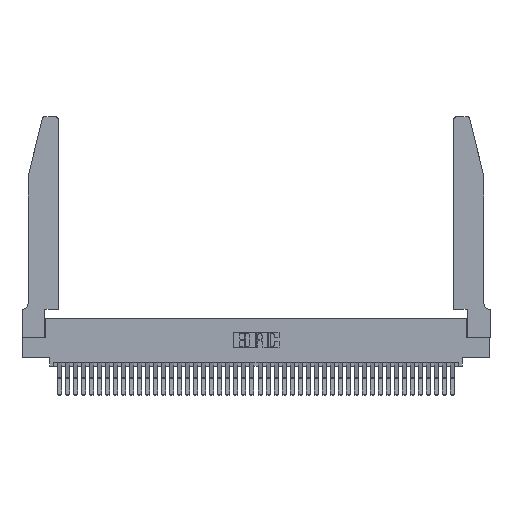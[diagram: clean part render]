
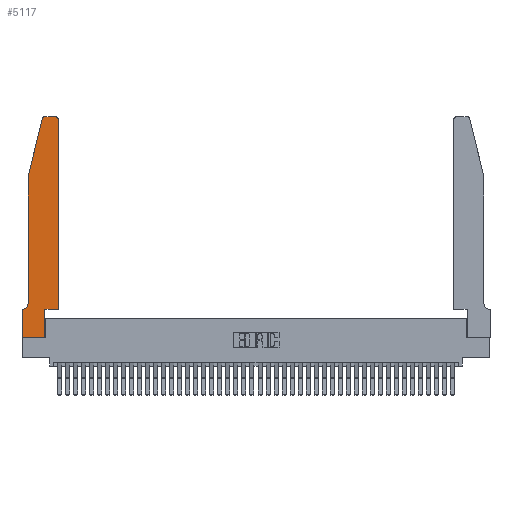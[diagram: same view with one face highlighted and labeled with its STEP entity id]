
A CAD part, top view. The second image highlights one B-rep face of the part: STEP entity #5117.
In plain terms, the highlighted planar face has unit normal (0, 0, 1).
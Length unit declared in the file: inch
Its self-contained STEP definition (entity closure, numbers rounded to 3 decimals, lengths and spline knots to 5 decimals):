
#58 = CARTESIAN_POINT ( 'NONE',  ( 0.0055, 0.42, 0.37 ) ) ;
#121 = EDGE_CURVE ( 'NONE', #27266, #37810, #22057, .T. ) ;
#180 = EDGE_CURVE ( 'NONE', #30962, #11434, #19940, .T. ) ;
#817 = DIRECTION ( 'NONE',  ( 1., 0., 0. ) ) ;
#1511 = ORIENTED_EDGE ( 'NONE', *, *, #180, .T. ) ;
#1961 = DIRECTION ( 'NONE',  ( 0., -1., 0. ) ) ;
#2182 = ORIENTED_EDGE ( 'NONE', *, *, #34164, .T. ) ;
#3515 = DIRECTION ( 'NONE',  ( -1., 0., 0. ) ) ;
#4806 = VECTOR ( 'NONE', #10750, 39.37008 ) ;
#5041 = LINE ( 'NONE', #36762, #21763 ) ;
#5117 = ADVANCED_FACE ( 'NONE', ( #43057 ), #40735, .T. ) ;
#5299 = ORIENTED_EDGE ( 'NONE', *, *, #14203, .T. ) ;
#5382 = CARTESIAN_POINT ( 'NONE',  ( 0., 0., 0.37 ) ) ;
#5452 = AXIS2_PLACEMENT_3D ( 'NONE', #30753, #20902, #817 ) ;
#6016 = VERTEX_POINT ( 'NONE', #10846 ) ;
#6853 = CARTESIAN_POINT ( 'NONE',  ( 0.0755, 2., 0.37 ) ) ;
#6960 = DIRECTION ( 'NONE',  ( 0., 0., 1. ) ) ;
#7307 = VECTOR ( 'NONE', #1961, 39.37008 ) ;
#7710 = VERTEX_POINT ( 'NONE', #37057 ) ;
#7961 = EDGE_CURVE ( 'NONE', #31423, #30962, #41799, .T. ) ;
#9518 = VECTOR ( 'NONE', #15072, 39.37008 ) ;
#9630 = EDGE_CURVE ( 'NONE', #13893, #27266, #41413, .T. ) ;
#10364 = CARTESIAN_POINT ( 'NONE',  ( 0., 0.35, 0.37 ) ) ;
#10545 = ORIENTED_EDGE ( 'NONE', *, *, #7961, .T. ) ;
#10750 = DIRECTION ( 'NONE',  ( 0., 1., 0. ) ) ;
#10846 = CARTESIAN_POINT ( 'NONE',  ( 0.0055, 0.35, 0.37 ) ) ;
#11434 = VERTEX_POINT ( 'NONE', #24727 ) ;
#11693 = CARTESIAN_POINT ( 'NONE',  ( 0.2865, 0., 0.37 ) ) ;
#11729 = CARTESIAN_POINT ( 'NONE',  ( 0.0755, 0.35, 0.37 ) ) ;
#11989 = DIRECTION ( 'NONE',  ( 0., 0., 1. ) ) ;
#12256 = EDGE_LOOP ( 'NONE', ( #35621, #10545, #1511, #38137, #2182, #19437, #5299, #24177, #23634, #24632, #42193, #20119 ) ) ;
#12315 = AXIS2_PLACEMENT_3D ( 'NONE', #58, #23558, #3515 ) ;
#12738 = EDGE_CURVE ( 'NONE', #6016, #31479, #36079, .T. ) ;
#13349 = VECTOR ( 'NONE', #40466, 39.37008 ) ;
#13879 = VECTOR ( 'NONE', #42275, 39.37008 ) ;
#13893 = VERTEX_POINT ( 'NONE', #40827 ) ;
#14203 = EDGE_CURVE ( 'NONE', #31479, #13893, #25088, .T. ) ;
#15072 = DIRECTION ( 'NONE',  ( -1., 0., 0. ) ) ;
#16356 = EDGE_CURVE ( 'NONE', #7710, #25746, #40161, .T. ) ;
#16581 = DIRECTION ( 'NONE',  ( 0., 1., 0. ) ) ;
#16738 = CARTESIAN_POINT ( 'NONE',  ( 0.284, 2.75, 0.37 ) ) ;
#16876 = DIRECTION ( 'NONE',  ( -0.239, -0.971, 0. ) ) ;
#19437 = ORIENTED_EDGE ( 'NONE', *, *, #12738, .T. ) ;
#19570 = CARTESIAN_POINT ( 'NONE',  ( 0.0755, 2., 0.37 ) ) ;
#19940 = LINE ( 'NONE', #6853, #27760 ) ;
#19994 = CARTESIAN_POINT ( 'NONE',  ( 0.2865, 0.35, 0.37 ) ) ;
#20119 = ORIENTED_EDGE ( 'NONE', *, *, #23086, .T. ) ;
#20258 = VERTEX_POINT ( 'NONE', #35682 ) ;
#20635 = CARTESIAN_POINT ( 'NONE',  ( 0.4505, 0.35, 0.37 ) ) ;
#20902 = DIRECTION ( 'NONE',  ( 0., 0., 1. ) ) ;
#21763 = VECTOR ( 'NONE', #40054, 39.37008 ) ;
#21783 = AXIS2_PLACEMENT_3D ( 'NONE', #31946, #11989, #35292 ) ;
#22057 = LINE ( 'NONE', #19994, #30847 ) ;
#22251 = VECTOR ( 'NONE', #26157, 39.37008 ) ;
#22292 = LINE ( 'NONE', #20635, #13349 ) ;
#23086 = EDGE_CURVE ( 'NONE', #25746, #31491, #33403, .T. ) ;
#23558 = DIRECTION ( 'NONE',  ( 0., 0., -1. ) ) ;
#23634 = ORIENTED_EDGE ( 'NONE', *, *, #121, .T. ) ;
#24177 = ORIENTED_EDGE ( 'NONE', *, *, #9630, .T. ) ;
#24349 = LINE ( 'NONE', #19570, #22251 ) ;
#24632 = ORIENTED_EDGE ( 'NONE', *, *, #37028, .T. ) ;
#24727 = CARTESIAN_POINT ( 'NONE',  ( 0.0755, 2., 0.37 ) ) ;
#25088 = LINE ( 'NONE', #5382, #7307 ) ;
#25746 = VERTEX_POINT ( 'NONE', #30775 ) ;
#26157 = DIRECTION ( 'NONE',  ( 0., -1., 0. ) ) ;
#26604 = CARTESIAN_POINT ( 'NONE',  ( 0.25487, 2.72718, 0.37 ) ) ;
#26967 = CARTESIAN_POINT ( 'NONE',  ( 0.4205, 2.72, 0.37 ) ) ;
#27266 = VERTEX_POINT ( 'NONE', #11693 ) ;
#27760 = VECTOR ( 'NONE', #16876, 39.37008 ) ;
#29004 = CARTESIAN_POINT ( 'NONE',  ( 0., 0., 0.37 ) ) ;
#30259 = DIRECTION ( 'NONE',  ( 1., 0., 0. ) ) ;
#30437 = CARTESIAN_POINT ( 'NONE',  ( 0.4205, 2.75, 0.37 ) ) ;
#30753 = CARTESIAN_POINT ( 'NONE',  ( 0., 0.35, 0.37 ) ) ;
#30775 = CARTESIAN_POINT ( 'NONE',  ( 0.4505, 2.72, 0.37 ) ) ;
#30847 = VECTOR ( 'NONE', #16581, 39.37008 ) ;
#30962 = VERTEX_POINT ( 'NONE', #26604 ) ;
#31423 = VERTEX_POINT ( 'NONE', #16738 ) ;
#31446 = CARTESIAN_POINT ( 'NONE',  ( 0.2865, 0.35, 0.37 ) ) ;
#31479 = VERTEX_POINT ( 'NONE', #10364 ) ;
#31491 = VERTEX_POINT ( 'NONE', #30437 ) ;
#31946 = CARTESIAN_POINT ( 'NONE',  ( 0.284, 2.72, 0.37 ) ) ;
#32147 = AXIS2_PLACEMENT_3D ( 'NONE', #26967, #6960, #30259 ) ;
#33403 = CIRCLE ( 'NONE', #32147, 0.03 ) ;
#33516 = EDGE_CURVE ( 'NONE', #31491, #31423, #5041, .T. ) ;
#34026 = CARTESIAN_POINT ( 'NONE',  ( 0.4505, 0.35, 0.37 ) ) ;
#34164 = EDGE_CURVE ( 'NONE', #20258, #6016, #40841, .T. ) ;
#35292 = DIRECTION ( 'NONE',  ( 1., 0., 0. ) ) ;
#35621 = ORIENTED_EDGE ( 'NONE', *, *, #33516, .T. ) ;
#35682 = CARTESIAN_POINT ( 'NONE',  ( 0.0755, 0.42, 0.37 ) ) ;
#36079 = LINE ( 'NONE', #11729, #9518 ) ;
#36762 = CARTESIAN_POINT ( 'NONE',  ( 0.2605, 2.75, 0.37 ) ) ;
#37028 = EDGE_CURVE ( 'NONE', #37810, #7710, #22292, .T. ) ;
#37057 = CARTESIAN_POINT ( 'NONE',  ( 0.4505, 0.35, 0.37 ) ) ;
#37462 = EDGE_CURVE ( 'NONE', #11434, #20258, #24349, .T. ) ;
#37810 = VERTEX_POINT ( 'NONE', #31446 ) ;
#38137 = ORIENTED_EDGE ( 'NONE', *, *, #37462, .T. ) ;
#40054 = DIRECTION ( 'NONE',  ( -1., 0., 0. ) ) ;
#40161 = LINE ( 'NONE', #34026, #4806 ) ;
#40466 = DIRECTION ( 'NONE',  ( 1., 0., 0. ) ) ;
#40735 = PLANE ( 'NONE',  #5452 ) ;
#40827 = CARTESIAN_POINT ( 'NONE',  ( 0., 0., 0.37 ) ) ;
#40841 = CIRCLE ( 'NONE', #12315, 0.07 ) ;
#41413 = LINE ( 'NONE', #29004, #13879 ) ;
#41799 = CIRCLE ( 'NONE', #21783, 0.03 ) ;
#42193 = ORIENTED_EDGE ( 'NONE', *, *, #16356, .T. ) ;
#42275 = DIRECTION ( 'NONE',  ( 1., 0., 0. ) ) ;
#43057 = FACE_OUTER_BOUND ( 'NONE', #12256, .T. ) ;
